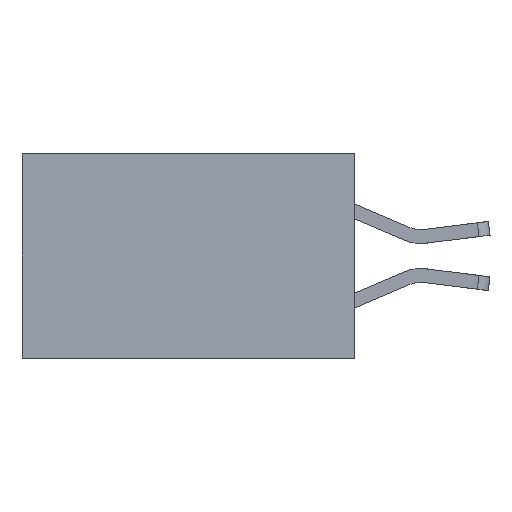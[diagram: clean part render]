
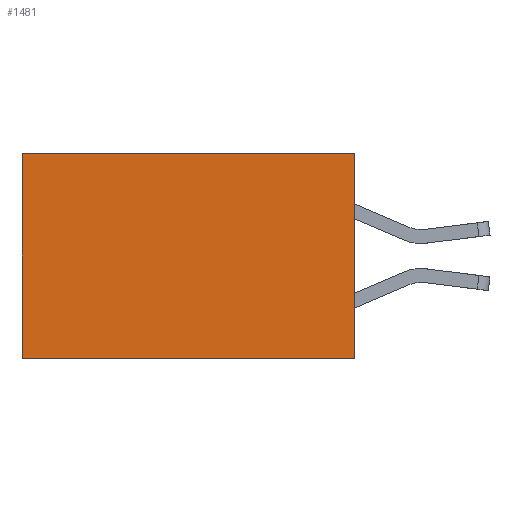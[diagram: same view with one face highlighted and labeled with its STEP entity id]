
A CAD part, left-side view. The second image highlights one B-rep face of the part: STEP entity #1481.
In plain terms, the highlighted planar face has unit normal (-1, 0, 0).
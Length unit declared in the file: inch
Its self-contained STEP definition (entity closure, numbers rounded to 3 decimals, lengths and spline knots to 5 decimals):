
#113 = DIRECTION ( 'NONE',  ( 0., 0., -1. ) ) ;
#211 = LINE ( 'NONE', #12984, #13185 ) ;
#582 = EDGE_CURVE ( 'NONE', #6503, #12372, #8661, .T. ) ;
#713 = EDGE_LOOP ( 'NONE', ( #5986, #12866, #9259, #9652 ) ) ;
#755 = EDGE_CURVE ( 'NONE', #3640, #3130, #12219, .T. ) ;
#1295 = PLANE ( 'NONE',  #2176 ) ;
#1481 = ADVANCED_FACE ( 'NONE', ( #11089 ), #1295, .F. ) ;
#2176 = AXIS2_PLACEMENT_3D ( 'NONE', #2664, #5032, #8040 ) ;
#2664 = CARTESIAN_POINT ( 'NONE',  ( 0.298, 0., 0. ) ) ;
#3130 = VERTEX_POINT ( 'NONE', #10010 ) ;
#3461 = VECTOR ( 'NONE', #9484, 39.37008 ) ;
#3640 = VERTEX_POINT ( 'NONE', #11577 ) ;
#3818 = DIRECTION ( 'NONE',  ( 0., 1., 0. ) ) ;
#4956 = EDGE_CURVE ( 'NONE', #3640, #6503, #211, .T. ) ;
#5032 = DIRECTION ( 'NONE',  ( 1., 0., 0. ) ) ;
#5215 = CARTESIAN_POINT ( 'NONE',  ( 0.298, 0.6, -0.37 ) ) ;
#5817 = DIRECTION ( 'NONE',  ( 0., 1., 0. ) ) ;
#5830 = EDGE_CURVE ( 'NONE', #3130, #12372, #6162, .T. ) ;
#5837 = VECTOR ( 'NONE', #3818, 39.37008 ) ;
#5986 = ORIENTED_EDGE ( 'NONE', *, *, #582, .T. ) ;
#6162 = LINE ( 'NONE', #9057, #5837 ) ;
#6340 = VECTOR ( 'NONE', #113, 39.37008 ) ;
#6479 = CARTESIAN_POINT ( 'NONE',  ( 0.298, 0., 0. ) ) ;
#6503 = VERTEX_POINT ( 'NONE', #9287 ) ;
#8040 = DIRECTION ( 'NONE',  ( 0., 0., -1. ) ) ;
#8396 = CARTESIAN_POINT ( 'NONE',  ( 0.298, 0.6, 0. ) ) ;
#8661 = LINE ( 'NONE', #8396, #3461 ) ;
#9057 = CARTESIAN_POINT ( 'NONE',  ( 0.298, 0., -0.37 ) ) ;
#9259 = ORIENTED_EDGE ( 'NONE', *, *, #755, .F. ) ;
#9287 = CARTESIAN_POINT ( 'NONE',  ( 0.298, 0.6, 0. ) ) ;
#9484 = DIRECTION ( 'NONE',  ( 0., 0., -1. ) ) ;
#9652 = ORIENTED_EDGE ( 'NONE', *, *, #4956, .T. ) ;
#10010 = CARTESIAN_POINT ( 'NONE',  ( 0.298, 0., -0.37 ) ) ;
#11089 = FACE_OUTER_BOUND ( 'NONE', #713, .T. ) ;
#11577 = CARTESIAN_POINT ( 'NONE',  ( 0.298, 0., 0. ) ) ;
#12219 = LINE ( 'NONE', #6479, #6340 ) ;
#12372 = VERTEX_POINT ( 'NONE', #5215 ) ;
#12866 = ORIENTED_EDGE ( 'NONE', *, *, #5830, .F. ) ;
#12984 = CARTESIAN_POINT ( 'NONE',  ( 0.298, 0., 0. ) ) ;
#13185 = VECTOR ( 'NONE', #5817, 39.37008 ) ;
